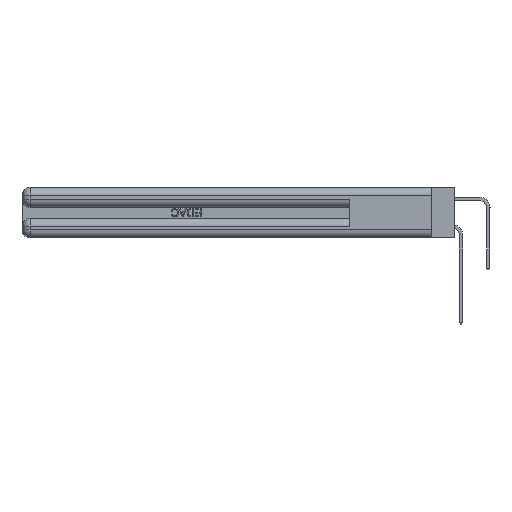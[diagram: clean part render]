
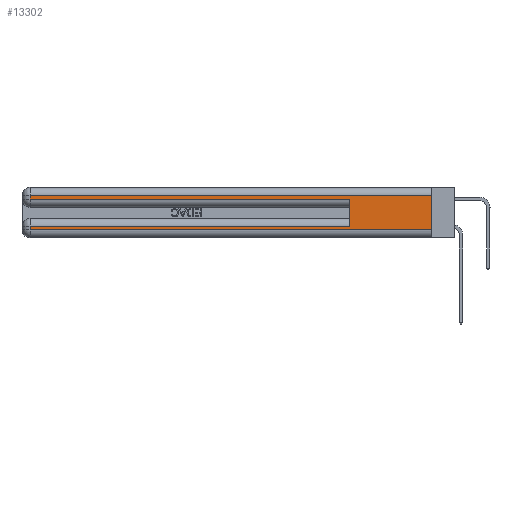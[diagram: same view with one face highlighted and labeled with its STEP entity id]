
A CAD part, left-side view. The second image highlights one B-rep face of the part: STEP entity #13302.
In plain terms, the highlighted planar face has unit normal (-1, 0, 0).
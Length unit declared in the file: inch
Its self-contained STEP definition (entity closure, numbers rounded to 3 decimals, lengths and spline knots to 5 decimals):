
#76 = EDGE_CURVE ( 'NONE', #12431, #46523, #38678, .T. ) ;
#448 = VECTOR ( 'NONE', #25655, 39.37008 ) ;
#514 = CARTESIAN_POINT ( 'NONE',  ( 0., 2.94, 0.285 ) ) ;
#677 = EDGE_CURVE ( 'NONE', #23786, #46523, #10857, .T. ) ;
#1178 = VERTEX_POINT ( 'NONE', #514 ) ;
#1409 = EDGE_CURVE ( 'NONE', #11911, #23786, #34844, .T. ) ;
#1520 = EDGE_CURVE ( 'NONE', #1178, #18982, #6480, .T. ) ;
#2168 = CARTESIAN_POINT ( 'NONE',  ( 0., 2.94, 0.37 ) ) ;
#2382 = CARTESIAN_POINT ( 'NONE',  ( 0., 0., 0.31 ) ) ;
#3276 = EDGE_CURVE ( 'NONE', #36572, #1178, #37708, .T. ) ;
#4771 = VECTOR ( 'NONE', #18410, 39.37008 ) ;
#5093 = ORIENTED_EDGE ( 'NONE', *, *, #76, .F. ) ;
#5443 = DIRECTION ( 'NONE',  ( 1., 0., 0. ) ) ;
#5540 = CARTESIAN_POINT ( 'NONE',  ( 0., 0.6, 0.145 ) ) ;
#6480 = LINE ( 'NONE', #39834, #48994 ) ;
#6578 = CARTESIAN_POINT ( 'NONE',  ( 0., 0.6, 0.285 ) ) ;
#7187 = DIRECTION ( 'NONE',  ( 0., 1., 0. ) ) ;
#7778 = ORIENTED_EDGE ( 'NONE', *, *, #1409, .T. ) ;
#8171 = CARTESIAN_POINT ( 'NONE',  ( 0., 0., 0.37 ) ) ;
#8935 = LINE ( 'NONE', #26805, #41659 ) ;
#10505 = EDGE_CURVE ( 'NONE', #23748, #11911, #8935, .T. ) ;
#10857 = LINE ( 'NONE', #45360, #448 ) ;
#11911 = VERTEX_POINT ( 'NONE', #16027 ) ;
#12431 = VERTEX_POINT ( 'NONE', #26851 ) ;
#13302 = ADVANCED_FACE ( 'NONE', ( #18948 ), #31793, .F. ) ;
#15909 = DIRECTION ( 'NONE',  ( 0., 0., -1. ) ) ;
#16027 = CARTESIAN_POINT ( 'NONE',  ( 0., 2.94, 0.085 ) ) ;
#16386 = EDGE_CURVE ( 'NONE', #23748, #18982, #22976, .T. ) ;
#16776 = DIRECTION ( 'NONE',  ( 0., 0., -1. ) ) ;
#18235 = CARTESIAN_POINT ( 'NONE',  ( 0., 0., 0.06 ) ) ;
#18410 = DIRECTION ( 'NONE',  ( 0., 0., -1. ) ) ;
#18948 = FACE_OUTER_BOUND ( 'NONE', #33001, .T. ) ;
#18982 = VERTEX_POINT ( 'NONE', #6578 ) ;
#20553 = ORIENTED_EDGE ( 'NONE', *, *, #1520, .T. ) ;
#22113 = DIRECTION ( 'NONE',  ( 0., 0., -1. ) ) ;
#22123 = LINE ( 'NONE', #2382, #45617 ) ;
#22976 = LINE ( 'NONE', #5540, #34691 ) ;
#23442 = AXIS2_PLACEMENT_3D ( 'NONE', #8171, #5443, #15909 ) ;
#23748 = VERTEX_POINT ( 'NONE', #46346 ) ;
#23786 = VERTEX_POINT ( 'NONE', #43235 ) ;
#25655 = DIRECTION ( 'NONE',  ( 0., -1., 0. ) ) ;
#26805 = CARTESIAN_POINT ( 'NONE',  ( 0., 0., 0.085 ) ) ;
#26851 = CARTESIAN_POINT ( 'NONE',  ( 0., 0., 0.31 ) ) ;
#27853 = CARTESIAN_POINT ( 'NONE',  ( 0., 2.94, 0.31 ) ) ;
#31793 = PLANE ( 'NONE',  #23442 ) ;
#33001 = EDGE_LOOP ( 'NONE', ( #5093, #36644, #49435, #20553, #36014, #41786, #7778, #48473 ) ) ;
#33079 = DIRECTION ( 'NONE',  ( 0., 0., 1. ) ) ;
#33618 = VECTOR ( 'NONE', #22113, 39.37008 ) ;
#34691 = VECTOR ( 'NONE', #33079, 39.37008 ) ;
#34844 = LINE ( 'NONE', #2168, #33618 ) ;
#36014 = ORIENTED_EDGE ( 'NONE', *, *, #16386, .F. ) ;
#36572 = VERTEX_POINT ( 'NONE', #27853 ) ;
#36644 = ORIENTED_EDGE ( 'NONE', *, *, #48320, .T. ) ;
#37658 = DIRECTION ( 'NONE',  ( 0., 1., 0. ) ) ;
#37708 = LINE ( 'NONE', #43907, #46362 ) ;
#38678 = LINE ( 'NONE', #42064, #4771 ) ;
#39834 = CARTESIAN_POINT ( 'NONE',  ( 0., 0., 0.285 ) ) ;
#41659 = VECTOR ( 'NONE', #7187, 39.37008 ) ;
#41786 = ORIENTED_EDGE ( 'NONE', *, *, #10505, .T. ) ;
#42064 = CARTESIAN_POINT ( 'NONE',  ( 0., 0., 0.37 ) ) ;
#43235 = CARTESIAN_POINT ( 'NONE',  ( 0., 2.94, 0.06 ) ) ;
#43907 = CARTESIAN_POINT ( 'NONE',  ( 0., 2.94, 0.37 ) ) ;
#45360 = CARTESIAN_POINT ( 'NONE',  ( 0., 0., 0.06 ) ) ;
#45617 = VECTOR ( 'NONE', #37658, 39.37008 ) ;
#46346 = CARTESIAN_POINT ( 'NONE',  ( 0., 0.6, 0.085 ) ) ;
#46362 = VECTOR ( 'NONE', #16776, 39.37008 ) ;
#46523 = VERTEX_POINT ( 'NONE', #18235 ) ;
#48320 = EDGE_CURVE ( 'NONE', #12431, #36572, #22123, .T. ) ;
#48473 = ORIENTED_EDGE ( 'NONE', *, *, #677, .T. ) ;
#48737 = DIRECTION ( 'NONE',  ( 0., -1., 0. ) ) ;
#48994 = VECTOR ( 'NONE', #48737, 39.37008 ) ;
#49435 = ORIENTED_EDGE ( 'NONE', *, *, #3276, .T. ) ;
